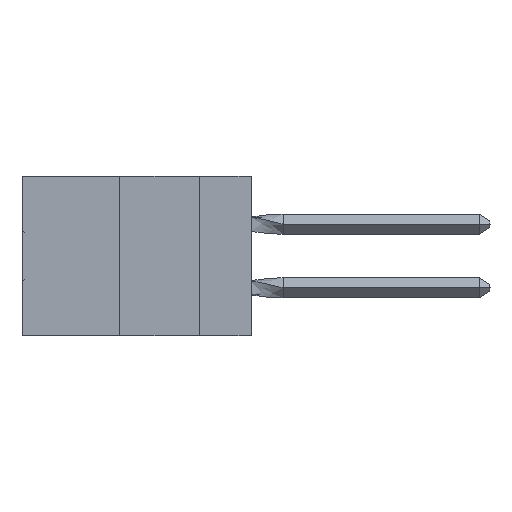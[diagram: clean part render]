
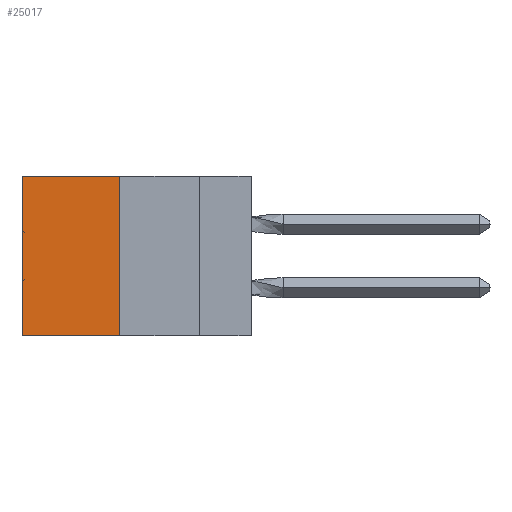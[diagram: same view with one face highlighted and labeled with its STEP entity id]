
A CAD part, left-side view. The second image highlights one B-rep face of the part: STEP entity #25017.
In plain terms, the highlighted planar face has unit normal (-1, 0, 0).
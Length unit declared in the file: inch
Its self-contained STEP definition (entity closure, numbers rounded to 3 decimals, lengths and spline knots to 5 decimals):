
#2024 = VECTOR ( 'NONE', #40925, 39.37008 ) ;
#2716 = DIRECTION ( 'NONE',  ( 0., 1., 0. ) ) ;
#3950 = VECTOR ( 'NONE', #2716, 39.37008 ) ;
#4705 = CARTESIAN_POINT ( 'NONE',  ( 0.305, 0.72, -0.5 ) ) ;
#4922 = DIRECTION ( 'NONE',  ( 0., 1., 0. ) ) ;
#6689 = ORIENTED_EDGE ( 'NONE', *, *, #33707, .T. ) ;
#6789 = LINE ( 'NONE', #14018, #2024 ) ;
#8503 = DIRECTION ( 'NONE',  ( 1., 0., 0. ) ) ;
#9033 = ORIENTED_EDGE ( 'NONE', *, *, #23979, .T. ) ;
#11763 = FACE_OUTER_BOUND ( 'NONE', #22527, .T. ) ;
#12160 = CARTESIAN_POINT ( 'NONE',  ( 0.305, 0.413, -0.5 ) ) ;
#13702 = ORIENTED_EDGE ( 'NONE', *, *, #48890, .F. ) ;
#14018 = CARTESIAN_POINT ( 'NONE',  ( 0.305, 0.72, -0.5 ) ) ;
#15366 = VECTOR ( 'NONE', #38021, 39.37008 ) ;
#16855 = VERTEX_POINT ( 'NONE', #35898 ) ;
#18278 = LINE ( 'NONE', #32665, #3950 ) ;
#18324 = LINE ( 'NONE', #22748, #15366 ) ;
#22527 = EDGE_LOOP ( 'NONE', ( #6689, #42840, #13702, #9033 ) ) ;
#22748 = CARTESIAN_POINT ( 'NONE',  ( 0.305, 0.413, -0.5 ) ) ;
#23341 = VERTEX_POINT ( 'NONE', #48612 ) ;
#23484 = PLANE ( 'NONE',  #31779 ) ;
#23496 = CARTESIAN_POINT ( 'NONE',  ( 0.305, 0.413, 0. ) ) ;
#23979 = EDGE_CURVE ( 'NONE', #45122, #16855, #39852, .T. ) ;
#25017 = ADVANCED_FACE ( 'NONE', ( #11763 ), #23484, .F. ) ;
#27440 = CARTESIAN_POINT ( 'NONE',  ( 0.305, 0.413, 0. ) ) ;
#31779 = AXIS2_PLACEMENT_3D ( 'NONE', #12160, #8503, #38734 ) ;
#32665 = CARTESIAN_POINT ( 'NONE',  ( 0.305, 0.413, -0.5 ) ) ;
#33707 = EDGE_CURVE ( 'NONE', #16855, #46320, #6789, .T. ) ;
#35898 = CARTESIAN_POINT ( 'NONE',  ( 0.305, 0.72, 0. ) ) ;
#38021 = DIRECTION ( 'NONE',  ( 0., 0., -1. ) ) ;
#38734 = DIRECTION ( 'NONE',  ( 0., 0., -1. ) ) ;
#39852 = LINE ( 'NONE', #27440, #42823 ) ;
#40606 = EDGE_CURVE ( 'NONE', #23341, #46320, #18278, .T. ) ;
#40925 = DIRECTION ( 'NONE',  ( 0., 0., -1. ) ) ;
#42823 = VECTOR ( 'NONE', #4922, 39.37008 ) ;
#42840 = ORIENTED_EDGE ( 'NONE', *, *, #40606, .F. ) ;
#45122 = VERTEX_POINT ( 'NONE', #23496 ) ;
#46320 = VERTEX_POINT ( 'NONE', #4705 ) ;
#48612 = CARTESIAN_POINT ( 'NONE',  ( 0.305, 0.413, -0.5 ) ) ;
#48890 = EDGE_CURVE ( 'NONE', #45122, #23341, #18324, .T. ) ;
